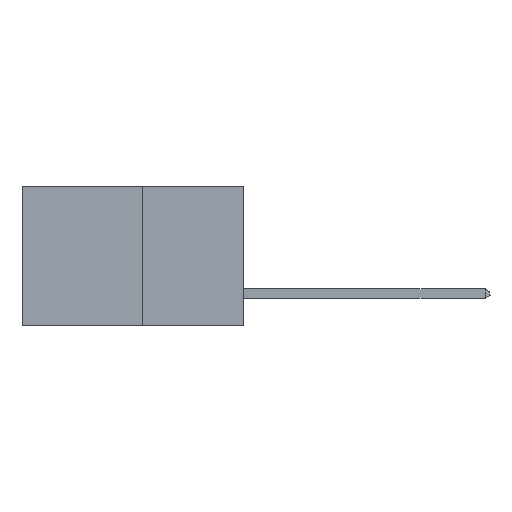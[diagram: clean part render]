
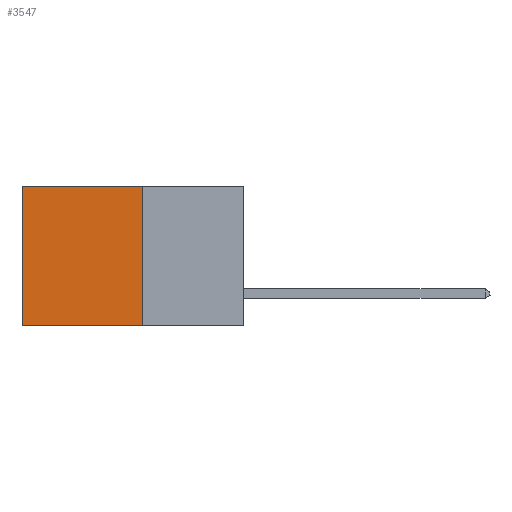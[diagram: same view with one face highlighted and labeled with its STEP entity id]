
A CAD part, left-side view. The second image highlights one B-rep face of the part: STEP entity #3547.
In plain terms, the highlighted planar face has unit normal (-1, 0, 0).
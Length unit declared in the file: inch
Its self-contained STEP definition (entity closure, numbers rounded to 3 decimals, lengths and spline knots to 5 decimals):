
#30 = CARTESIAN_POINT ( 'NONE',  ( 0.277, 0.27, -0.37 ) ) ;
#74 = LINE ( 'NONE', #9399, #5906 ) ;
#549 = DIRECTION ( 'NONE',  ( 0., 0., -1. ) ) ;
#731 = EDGE_CURVE ( 'NONE', #8088, #9814, #8349, .T. ) ;
#1060 = CARTESIAN_POINT ( 'NONE',  ( 0.277, 0.27, -0.37 ) ) ;
#1068 = DIRECTION ( 'NONE',  ( 1., 0., 0. ) ) ;
#1084 = DIRECTION ( 'NONE',  ( 0., 0., -1. ) ) ;
#1915 = EDGE_LOOP ( 'NONE', ( #7073, #5483, #3831, #4197 ) ) ;
#1979 = VECTOR ( 'NONE', #4879, 39.37008 ) ;
#2033 = VERTEX_POINT ( 'NONE', #4606 ) ;
#2126 = CARTESIAN_POINT ( 'NONE',  ( 0.277, 0.59, -0.37 ) ) ;
#3547 = ADVANCED_FACE ( 'NONE', ( #5544 ), #8298, .F. ) ;
#3831 = ORIENTED_EDGE ( 'NONE', *, *, #6846, .F. ) ;
#3943 = LINE ( 'NONE', #8032, #7693 ) ;
#4197 = ORIENTED_EDGE ( 'NONE', *, *, #8522, .T. ) ;
#4336 = VECTOR ( 'NONE', #9496, 39.37008 ) ;
#4539 = EDGE_CURVE ( 'NONE', #2033, #9814, #7858, .T. ) ;
#4606 = CARTESIAN_POINT ( 'NONE',  ( 0.277, 0.59, 0. ) ) ;
#4879 = DIRECTION ( 'NONE',  ( 0., 0., -1. ) ) ;
#4971 = AXIS2_PLACEMENT_3D ( 'NONE', #1060, #1068, #1084 ) ;
#5483 = ORIENTED_EDGE ( 'NONE', *, *, #731, .F. ) ;
#5544 = FACE_OUTER_BOUND ( 'NONE', #1915, .T. ) ;
#5906 = VECTOR ( 'NONE', #9518, 39.37008 ) ;
#6846 = EDGE_CURVE ( 'NONE', #6940, #8088, #3943, .T. ) ;
#6940 = VERTEX_POINT ( 'NONE', #9975 ) ;
#7073 = ORIENTED_EDGE ( 'NONE', *, *, #4539, .T. ) ;
#7693 = VECTOR ( 'NONE', #549, 39.37008 ) ;
#7858 = LINE ( 'NONE', #9289, #1979 ) ;
#8032 = CARTESIAN_POINT ( 'NONE',  ( 0.277, 0.27, -0.37 ) ) ;
#8088 = VERTEX_POINT ( 'NONE', #30 ) ;
#8298 = PLANE ( 'NONE',  #4971 ) ;
#8349 = LINE ( 'NONE', #8798, #4336 ) ;
#8522 = EDGE_CURVE ( 'NONE', #6940, #2033, #74, .T. ) ;
#8798 = CARTESIAN_POINT ( 'NONE',  ( 0.277, 0.27, -0.37 ) ) ;
#9289 = CARTESIAN_POINT ( 'NONE',  ( 0.277, 0.59, -0.37 ) ) ;
#9399 = CARTESIAN_POINT ( 'NONE',  ( 0.277, 0.27, 0. ) ) ;
#9496 = DIRECTION ( 'NONE',  ( 0., 1., 0. ) ) ;
#9518 = DIRECTION ( 'NONE',  ( 0., 1., 0. ) ) ;
#9814 = VERTEX_POINT ( 'NONE', #2126 ) ;
#9975 = CARTESIAN_POINT ( 'NONE',  ( 0.277, 0.27, 0. ) ) ;
